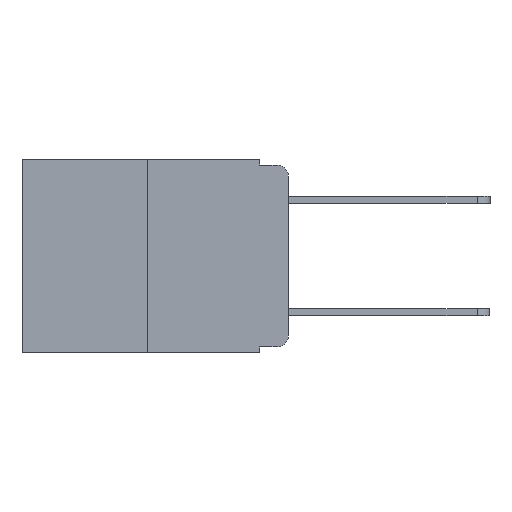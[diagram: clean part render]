
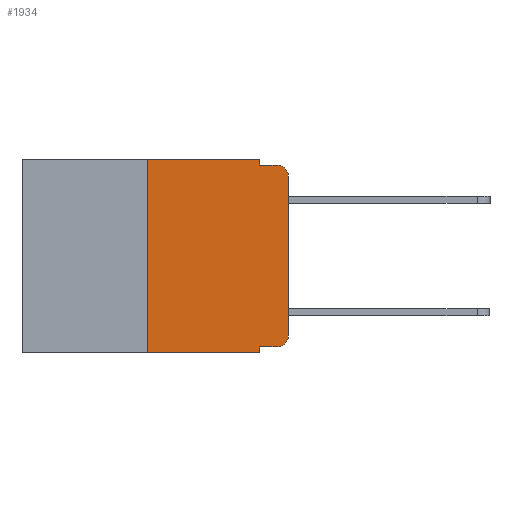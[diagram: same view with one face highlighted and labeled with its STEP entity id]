
A CAD part, left-side view. The second image highlights one B-rep face of the part: STEP entity #1934.
In plain terms, the highlighted planar face has unit normal (-1, 0, 0).
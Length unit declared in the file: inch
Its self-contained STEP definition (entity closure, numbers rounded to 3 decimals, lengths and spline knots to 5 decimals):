
#251 = CARTESIAN_POINT ( 'NONE',  ( 0., 0., 0. ) ) ;
#407 = DIRECTION ( 'NONE',  ( 0., 0., -1. ) ) ;
#574 = VECTOR ( 'NONE', #10744, 39.37008 ) ;
#784 = VERTEX_POINT ( 'NONE', #10185 ) ;
#1188 = CARTESIAN_POINT ( 'NONE',  ( 0., 0.051, -0.333 ) ) ;
#1934 = ADVANCED_FACE ( 'NONE', ( #8375 ), #17135, .F. ) ;
#2207 = ORIENTED_EDGE ( 'NONE', *, *, #7309, .F. ) ;
#2465 = ORIENTED_EDGE ( 'NONE', *, *, #15544, .F. ) ;
#2608 = LINE ( 'NONE', #2837, #6717 ) ;
#2837 = CARTESIAN_POINT ( 'NONE',  ( 0., 0.051, -0.01 ) ) ;
#2874 = VECTOR ( 'NONE', #17253, 39.37008 ) ;
#3325 = DIRECTION ( 'NONE',  ( 0., 0., 1. ) ) ;
#3330 = VERTEX_POINT ( 'NONE', #16282 ) ;
#3412 = ORIENTED_EDGE ( 'NONE', *, *, #3645, .F. ) ;
#3614 = ORIENTED_EDGE ( 'NONE', *, *, #6381, .F. ) ;
#3645 = EDGE_CURVE ( 'NONE', #8416, #9156, #13912, .T. ) ;
#3748 = AXIS2_PLACEMENT_3D ( 'NONE', #6657, #15725, #8036 ) ;
#3887 = LINE ( 'NONE', #251, #13210 ) ;
#3931 = AXIS2_PLACEMENT_3D ( 'NONE', #11055, #13679, #12035 ) ;
#4148 = DIRECTION ( 'NONE',  ( -1., 0., 0. ) ) ;
#4203 = ORIENTED_EDGE ( 'NONE', *, *, #9921, .T. ) ;
#4239 = ORIENTED_EDGE ( 'NONE', *, *, #11093, .T. ) ;
#4270 = EDGE_LOOP ( 'NONE', ( #4203, #11700, #2207, #3614, #2465, #3412, #7473, #16728, #13155, #4239 ) ) ;
#4435 = LINE ( 'NONE', #1188, #574 ) ;
#5314 = CARTESIAN_POINT ( 'NONE',  ( 0., 0.473, 0. ) ) ;
#5684 = EDGE_CURVE ( 'NONE', #8416, #13540, #13062, .T. ) ;
#6121 = CARTESIAN_POINT ( 'NONE',  ( 0., 0.051, 0. ) ) ;
#6145 = VECTOR ( 'NONE', #13709, 39.37008 ) ;
#6381 = EDGE_CURVE ( 'NONE', #8909, #7984, #17057, .T. ) ;
#6433 = CARTESIAN_POINT ( 'NONE',  ( 0., 0.051, -0.333 ) ) ;
#6657 = CARTESIAN_POINT ( 'NONE',  ( 0., 0.02, -0.313 ) ) ;
#6701 = DIRECTION ( 'NONE',  ( 0., -1., 0. ) ) ;
#6717 = VECTOR ( 'NONE', #14744, 39.37008 ) ;
#7309 = EDGE_CURVE ( 'NONE', #7984, #784, #2608, .T. ) ;
#7473 = ORIENTED_EDGE ( 'NONE', *, *, #5684, .T. ) ;
#7570 = LINE ( 'NONE', #6121, #14427 ) ;
#7984 = VERTEX_POINT ( 'NONE', #10772 ) ;
#8036 = DIRECTION ( 'NONE',  ( 0., 0., -1. ) ) ;
#8338 = CARTESIAN_POINT ( 'NONE',  ( 0., 0.473, -0.343 ) ) ;
#8375 = FACE_OUTER_BOUND ( 'NONE', #4270, .T. ) ;
#8416 = VERTEX_POINT ( 'NONE', #16826 ) ;
#8661 = VERTEX_POINT ( 'NONE', #15993 ) ;
#8909 = VERTEX_POINT ( 'NONE', #12707 ) ;
#9077 = EDGE_CURVE ( 'NONE', #13953, #784, #14399, .T. ) ;
#9156 = VERTEX_POINT ( 'NONE', #13517 ) ;
#9591 = VERTEX_POINT ( 'NONE', #6433 ) ;
#9921 = EDGE_CURVE ( 'NONE', #8661, #13953, #3887, .T. ) ;
#10185 = CARTESIAN_POINT ( 'NONE',  ( 0., 0.02, -0.01 ) ) ;
#10213 = AXIS2_PLACEMENT_3D ( 'NONE', #12125, #4148, #13414 ) ;
#10744 = DIRECTION ( 'NONE',  ( 0., -1., 0. ) ) ;
#10772 = CARTESIAN_POINT ( 'NONE',  ( 0., 0.051, -0.01 ) ) ;
#11055 = CARTESIAN_POINT ( 'NONE',  ( 0., 0.473, 0. ) ) ;
#11093 = EDGE_CURVE ( 'NONE', #3330, #8661, #12569, .T. ) ;
#11219 = CARTESIAN_POINT ( 'NONE',  ( 0., 0.051, 0. ) ) ;
#11700 = ORIENTED_EDGE ( 'NONE', *, *, #9077, .T. ) ;
#11993 = EDGE_CURVE ( 'NONE', #9591, #3330, #4435, .T. ) ;
#12035 = DIRECTION ( 'NONE',  ( 0., 0., -1. ) ) ;
#12125 = CARTESIAN_POINT ( 'NONE',  ( 0., 0.02, -0.03 ) ) ;
#12546 = DIRECTION ( 'NONE',  ( 0., 0., -1. ) ) ;
#12569 = CIRCLE ( 'NONE', #3748, 0.02 ) ;
#12707 = CARTESIAN_POINT ( 'NONE',  ( 0., 0.051, 0. ) ) ;
#12988 = LINE ( 'NONE', #5314, #16761 ) ;
#13062 = LINE ( 'NONE', #8338, #2874 ) ;
#13139 = CARTESIAN_POINT ( 'NONE',  ( 0., 0., -0.03 ) ) ;
#13155 = ORIENTED_EDGE ( 'NONE', *, *, #11993, .T. ) ;
#13210 = VECTOR ( 'NONE', #3325, 39.37008 ) ;
#13414 = DIRECTION ( 'NONE',  ( 0., 0., -1. ) ) ;
#13517 = CARTESIAN_POINT ( 'NONE',  ( 0., 0.25, 0. ) ) ;
#13540 = VERTEX_POINT ( 'NONE', #14894 ) ;
#13679 = DIRECTION ( 'NONE',  ( 1., 0., 0. ) ) ;
#13695 = VECTOR ( 'NONE', #12546, 39.37008 ) ;
#13709 = DIRECTION ( 'NONE',  ( 0., 0., 1. ) ) ;
#13710 = EDGE_CURVE ( 'NONE', #9591, #13540, #7570, .T. ) ;
#13912 = LINE ( 'NONE', #16258, #6145 ) ;
#13953 = VERTEX_POINT ( 'NONE', #13139 ) ;
#14399 = CIRCLE ( 'NONE', #10213, 0.02 ) ;
#14427 = VECTOR ( 'NONE', #407, 39.37008 ) ;
#14744 = DIRECTION ( 'NONE',  ( 0., -1., 0. ) ) ;
#14894 = CARTESIAN_POINT ( 'NONE',  ( 0., 0.051, -0.343 ) ) ;
#15544 = EDGE_CURVE ( 'NONE', #9156, #8909, #12988, .T. ) ;
#15725 = DIRECTION ( 'NONE',  ( -1., 0., 0. ) ) ;
#15993 = CARTESIAN_POINT ( 'NONE',  ( 0., 0., -0.313 ) ) ;
#16258 = CARTESIAN_POINT ( 'NONE',  ( 0., 0.25, 0. ) ) ;
#16282 = CARTESIAN_POINT ( 'NONE',  ( 0., 0.02, -0.333 ) ) ;
#16728 = ORIENTED_EDGE ( 'NONE', *, *, #13710, .F. ) ;
#16761 = VECTOR ( 'NONE', #6701, 39.37008 ) ;
#16826 = CARTESIAN_POINT ( 'NONE',  ( 0., 0.25, -0.343 ) ) ;
#17057 = LINE ( 'NONE', #11219, #13695 ) ;
#17135 = PLANE ( 'NONE',  #3931 ) ;
#17253 = DIRECTION ( 'NONE',  ( 0., -1., 0. ) ) ;
